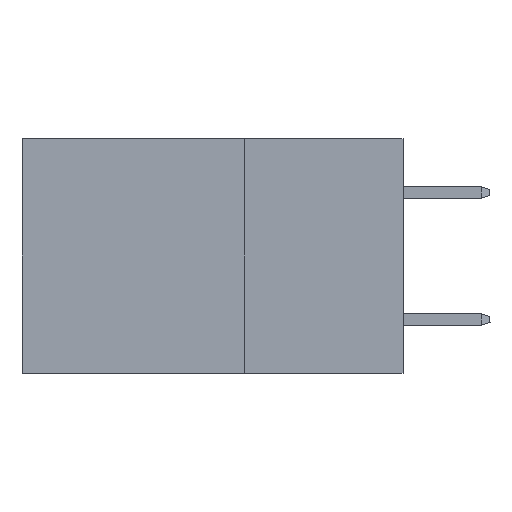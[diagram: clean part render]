
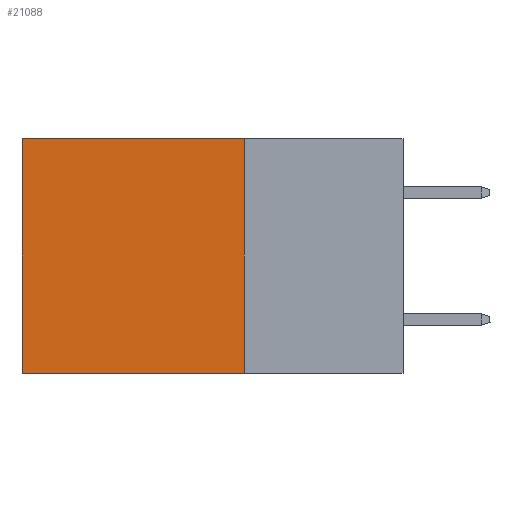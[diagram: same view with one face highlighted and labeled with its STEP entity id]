
A CAD part, left-side view. The second image highlights one B-rep face of the part: STEP entity #21088.
In plain terms, the highlighted planar face has unit normal (-1, 0, 0).
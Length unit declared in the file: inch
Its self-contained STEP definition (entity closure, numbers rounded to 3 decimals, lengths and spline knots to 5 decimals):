
#172 = LINE ( 'NONE', #2238, #10732 ) ;
#395 = DIRECTION ( 'NONE',  ( 0., 1., 0. ) ) ;
#2238 = CARTESIAN_POINT ( 'NONE',  ( 0.2875, 0.25, 0. ) ) ;
#3616 = CARTESIAN_POINT ( 'NONE',  ( 0.2875, 0.6, 0. ) ) ;
#4111 = VERTEX_POINT ( 'NONE', #16227 ) ;
#4322 = DIRECTION ( 'NONE',  ( 0., 0., -1. ) ) ;
#5300 = AXIS2_PLACEMENT_3D ( 'NONE', #18585, #6106, #16621 ) ;
#5869 = VERTEX_POINT ( 'NONE', #20485 ) ;
#6017 = EDGE_CURVE ( 'NONE', #11250, #4111, #172, .T. ) ;
#6106 = DIRECTION ( 'NONE',  ( 1., 0., 0. ) ) ;
#6685 = DIRECTION ( 'NONE',  ( 0., 1., 0. ) ) ;
#8387 = ORIENTED_EDGE ( 'NONE', *, *, #17821, .T. ) ;
#10732 = VECTOR ( 'NONE', #395, 39.37008 ) ;
#11250 = VERTEX_POINT ( 'NONE', #19602 ) ;
#11588 = FACE_OUTER_BOUND ( 'NONE', #21761, .T. ) ;
#12632 = DIRECTION ( 'NONE',  ( 0., 0., -1. ) ) ;
#12886 = CARTESIAN_POINT ( 'NONE',  ( 0.2875, 0.25, 0. ) ) ;
#13072 = EDGE_CURVE ( 'NONE', #22155, #5869, #13777, .T. ) ;
#13777 = LINE ( 'NONE', #22371, #18250 ) ;
#14278 = ORIENTED_EDGE ( 'NONE', *, *, #13072, .F. ) ;
#16227 = CARTESIAN_POINT ( 'NONE',  ( 0.2875, 0.6, 0. ) ) ;
#16245 = ORIENTED_EDGE ( 'NONE', *, *, #6017, .T. ) ;
#16570 = ORIENTED_EDGE ( 'NONE', *, *, #21728, .F. ) ;
#16621 = DIRECTION ( 'NONE',  ( 0., 0., -1. ) ) ;
#17821 = EDGE_CURVE ( 'NONE', #4111, #5869, #19752, .T. ) ;
#18250 = VECTOR ( 'NONE', #6685, 39.37008 ) ;
#18585 = CARTESIAN_POINT ( 'NONE',  ( 0.2875, 0.25, 0. ) ) ;
#18866 = VECTOR ( 'NONE', #4322, 39.37008 ) ;
#19424 = VECTOR ( 'NONE', #12632, 39.37008 ) ;
#19602 = CARTESIAN_POINT ( 'NONE',  ( 0.2875, 0.25, 0. ) ) ;
#19752 = LINE ( 'NONE', #3616, #19424 ) ;
#20130 = LINE ( 'NONE', #12886, #18866 ) ;
#20306 = PLANE ( 'NONE',  #5300 ) ;
#20485 = CARTESIAN_POINT ( 'NONE',  ( 0.2875, 0.6, -0.37 ) ) ;
#20702 = CARTESIAN_POINT ( 'NONE',  ( 0.2875, 0.25, -0.37 ) ) ;
#21088 = ADVANCED_FACE ( 'NONE', ( #11588 ), #20306, .F. ) ;
#21728 = EDGE_CURVE ( 'NONE', #11250, #22155, #20130, .T. ) ;
#21761 = EDGE_LOOP ( 'NONE', ( #8387, #14278, #16570, #16245 ) ) ;
#22155 = VERTEX_POINT ( 'NONE', #20702 ) ;
#22371 = CARTESIAN_POINT ( 'NONE',  ( 0.2875, 0.25, -0.37 ) ) ;
